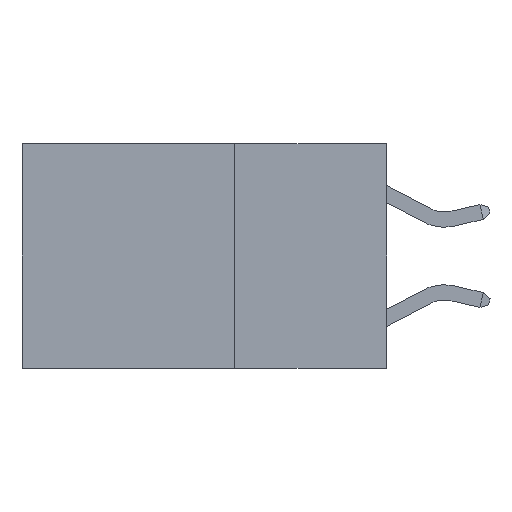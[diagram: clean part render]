
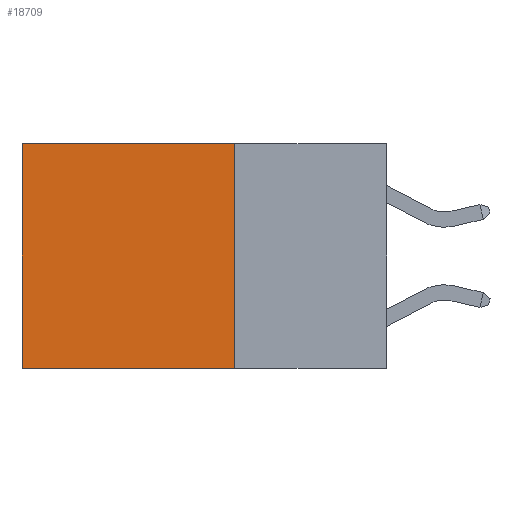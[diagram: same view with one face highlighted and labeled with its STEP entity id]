
A CAD part, left-side view. The second image highlights one B-rep face of the part: STEP entity #18709.
In plain terms, the highlighted planar face has unit normal (-1, 0, 0).
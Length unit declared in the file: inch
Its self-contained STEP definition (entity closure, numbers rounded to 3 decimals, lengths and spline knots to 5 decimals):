
#283 = CARTESIAN_POINT ( 'NONE',  ( 0.2625, 0.6, 0. ) ) ;
#514 = ORIENTED_EDGE ( 'NONE', *, *, #8724, .F. ) ;
#825 = DIRECTION ( 'NONE',  ( 0., 0., -1. ) ) ;
#1360 = CARTESIAN_POINT ( 'NONE',  ( 0.2625, 0.6, 0. ) ) ;
#1711 = CARTESIAN_POINT ( 'NONE',  ( 0.2625, 0.25, 0. ) ) ;
#1979 = VECTOR ( 'NONE', #10516, 39.37008 ) ;
#2899 = CARTESIAN_POINT ( 'NONE',  ( 0.2625, 0.6, -0.37 ) ) ;
#3353 = CARTESIAN_POINT ( 'NONE',  ( 0.2625, 0.25, 0. ) ) ;
#4552 = VECTOR ( 'NONE', #21239, 39.37008 ) ;
#4915 = VERTEX_POINT ( 'NONE', #20632 ) ;
#5963 = ORIENTED_EDGE ( 'NONE', *, *, #7749, .F. ) ;
#7566 = CARTESIAN_POINT ( 'NONE',  ( 0.2625, 0.25, -0.37 ) ) ;
#7749 = EDGE_CURVE ( 'NONE', #4915, #18064, #21823, .T. ) ;
#8596 = VECTOR ( 'NONE', #825, 39.37008 ) ;
#8724 = EDGE_CURVE ( 'NONE', #18064, #20573, #14062, .T. ) ;
#8756 = EDGE_LOOP ( 'NONE', ( #14470, #514, #5963, #15069 ) ) ;
#10516 = DIRECTION ( 'NONE',  ( 0., 1., 0. ) ) ;
#11200 = DIRECTION ( 'NONE',  ( 0., 1., 0. ) ) ;
#11433 = LINE ( 'NONE', #1711, #1979 ) ;
#11465 = CARTESIAN_POINT ( 'NONE',  ( 0.2625, 0.25, 0. ) ) ;
#12288 = DIRECTION ( 'NONE',  ( 0., 0., -1. ) ) ;
#12592 = VERTEX_POINT ( 'NONE', #1360 ) ;
#13952 = EDGE_CURVE ( 'NONE', #12592, #20573, #18538, .T. ) ;
#14062 = LINE ( 'NONE', #7566, #18071 ) ;
#14470 = ORIENTED_EDGE ( 'NONE', *, *, #13952, .T. ) ;
#15069 = ORIENTED_EDGE ( 'NONE', *, *, #21593, .T. ) ;
#15329 = AXIS2_PLACEMENT_3D ( 'NONE', #3353, #22563, #12288 ) ;
#15978 = CARTESIAN_POINT ( 'NONE',  ( 0.2625, 0.25, -0.37 ) ) ;
#18064 = VERTEX_POINT ( 'NONE', #15978 ) ;
#18071 = VECTOR ( 'NONE', #11200, 39.37008 ) ;
#18538 = LINE ( 'NONE', #283, #4552 ) ;
#18709 = ADVANCED_FACE ( 'NONE', ( #19078 ), #20858, .F. ) ;
#19078 = FACE_OUTER_BOUND ( 'NONE', #8756, .T. ) ;
#20573 = VERTEX_POINT ( 'NONE', #2899 ) ;
#20632 = CARTESIAN_POINT ( 'NONE',  ( 0.2625, 0.25, 0. ) ) ;
#20858 = PLANE ( 'NONE',  #15329 ) ;
#21239 = DIRECTION ( 'NONE',  ( 0., 0., -1. ) ) ;
#21593 = EDGE_CURVE ( 'NONE', #4915, #12592, #11433, .T. ) ;
#21823 = LINE ( 'NONE', #11465, #8596 ) ;
#22563 = DIRECTION ( 'NONE',  ( 1., 0., 0. ) ) ;
